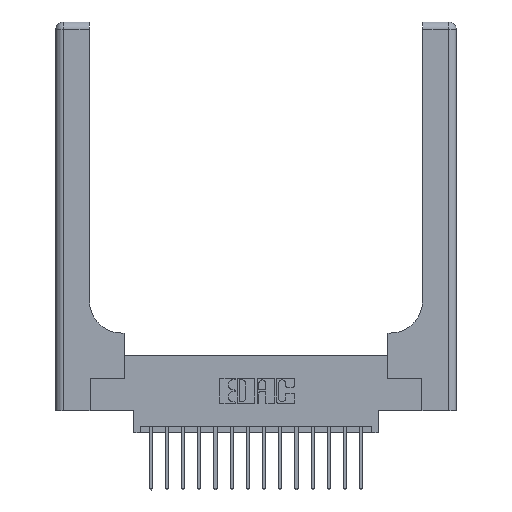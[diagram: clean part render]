
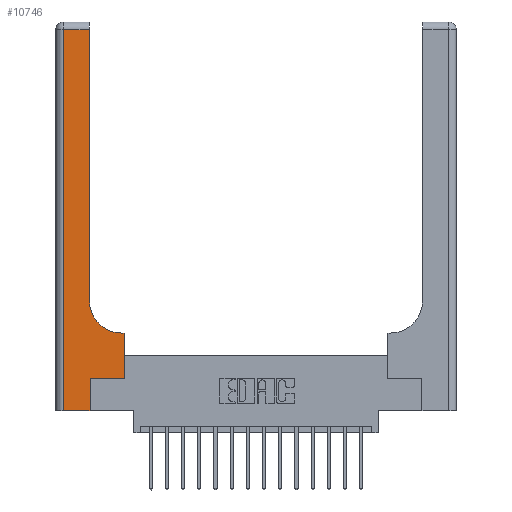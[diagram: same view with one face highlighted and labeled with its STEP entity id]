
A CAD part, top view. The second image highlights one B-rep face of the part: STEP entity #10746.
In plain terms, the highlighted planar face has unit normal (0, 0, 1).
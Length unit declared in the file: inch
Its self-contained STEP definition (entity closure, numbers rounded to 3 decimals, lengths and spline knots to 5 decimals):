
#49 = CARTESIAN_POINT ( 'NONE',  ( 0.06, 3., 0.37 ) ) ;
#151 = ORIENTED_EDGE ( 'NONE', *, *, #11037, .T. ) ;
#259 = LINE ( 'NONE', #7387, #7367 ) ;
#423 = CARTESIAN_POINT ( 'NONE',  ( 0.26, 2.94, 0.37 ) ) ;
#597 = LINE ( 'NONE', #11783, #11848 ) ;
#1410 = EDGE_CURVE ( 'NONE', #17213, #2887, #11189, .T. ) ;
#1603 = EDGE_CURVE ( 'NONE', #14179, #14640, #4391, .T. ) ;
#1753 = DIRECTION ( 'NONE',  ( -1., 0., 0. ) ) ;
#1934 = DIRECTION ( 'NONE',  ( 1., 0., 0. ) ) ;
#2081 = CARTESIAN_POINT ( 'NONE',  ( 0.06, 0., 0.37 ) ) ;
#2887 = VERTEX_POINT ( 'NONE', #10943 ) ;
#3300 = VECTOR ( 'NONE', #13908, 39.37008 ) ;
#3469 = ORIENTED_EDGE ( 'NONE', *, *, #1603, .T. ) ;
#3528 = CARTESIAN_POINT ( 'NONE',  ( 0.265, 0., 0.37 ) ) ;
#3656 = EDGE_LOOP ( 'NONE', ( #8706, #13283, #3469, #5011, #5250, #3946, #5719, #5957, #151 ) ) ;
#3802 = CARTESIAN_POINT ( 'NONE',  ( 0.51, 0.85, 0.37 ) ) ;
#3876 = VERTEX_POINT ( 'NONE', #10910 ) ;
#3946 = ORIENTED_EDGE ( 'NONE', *, *, #7716, .T. ) ;
#3948 = VECTOR ( 'NONE', #8976, 39.37008 ) ;
#4228 = DIRECTION ( 'NONE',  ( -1., 0., 0. ) ) ;
#4391 = LINE ( 'NONE', #49, #7697 ) ;
#4493 = AXIS2_PLACEMENT_3D ( 'NONE', #3802, #13614, #5221 ) ;
#5011 = ORIENTED_EDGE ( 'NONE', *, *, #11276, .T. ) ;
#5221 = DIRECTION ( 'NONE',  ( 1., 0., 0. ) ) ;
#5250 = ORIENTED_EDGE ( 'NONE', *, *, #1410, .T. ) ;
#5719 = ORIENTED_EDGE ( 'NONE', *, *, #7726, .T. ) ;
#5957 = ORIENTED_EDGE ( 'NONE', *, *, #18196, .T. ) ;
#5983 = CARTESIAN_POINT ( 'NONE',  ( 0., 3., 0.37 ) ) ;
#6732 = AXIS2_PLACEMENT_3D ( 'NONE', #5983, #15788, #7389 ) ;
#6751 = VECTOR ( 'NONE', #10928, 39.37008 ) ;
#6885 = VERTEX_POINT ( 'NONE', #10279 ) ;
#7297 = CARTESIAN_POINT ( 'NONE',  ( 0., 0., 0.37 ) ) ;
#7321 = PLANE ( 'NONE',  #6732 ) ;
#7367 = VECTOR ( 'NONE', #1753, 39.37008 ) ;
#7387 = CARTESIAN_POINT ( 'NONE',  ( 0., 2.94, 0.37 ) ) ;
#7389 = DIRECTION ( 'NONE',  ( -1., 0., 0. ) ) ;
#7697 = VECTOR ( 'NONE', #17817, 39.37008 ) ;
#7716 = EDGE_CURVE ( 'NONE', #2887, #3876, #597, .T. ) ;
#7726 = EDGE_CURVE ( 'NONE', #3876, #16120, #11396, .T. ) ;
#8358 = VERTEX_POINT ( 'NONE', #423 ) ;
#8706 = ORIENTED_EDGE ( 'NONE', *, *, #9185, .T. ) ;
#8719 = DIRECTION ( 'NONE',  ( 1., 0., 0. ) ) ;
#8976 = DIRECTION ( 'NONE',  ( 0., 1., 0. ) ) ;
#9185 = EDGE_CURVE ( 'NONE', #13386, #8358, #10896, .T. ) ;
#9306 = CIRCLE ( 'NONE', #4493, 0.25 ) ;
#9514 = LINE ( 'NONE', #7297, #16560 ) ;
#9520 = CARTESIAN_POINT ( 'NONE',  ( 0.26, 3., 0.37 ) ) ;
#9976 = FACE_OUTER_BOUND ( 'NONE', #3656, .T. ) ;
#10279 = CARTESIAN_POINT ( 'NONE',  ( 0.51, 0.6, 0.37 ) ) ;
#10746 = ADVANCED_FACE ( 'NONE', ( #9976 ), #7321, .F. ) ;
#10896 = LINE ( 'NONE', #9520, #6751 ) ;
#10910 = CARTESIAN_POINT ( 'NONE',  ( 0.528, 0.25, 0.37 ) ) ;
#10928 = DIRECTION ( 'NONE',  ( 0., 1., 0. ) ) ;
#10943 = CARTESIAN_POINT ( 'NONE',  ( 0.265, 0.25, 0.37 ) ) ;
#11037 = EDGE_CURVE ( 'NONE', #6885, #13386, #9306, .T. ) ;
#11189 = LINE ( 'NONE', #14123, #3300 ) ;
#11211 = CARTESIAN_POINT ( 'NONE',  ( 0.26, 0.6, 0.37 ) ) ;
#11276 = EDGE_CURVE ( 'NONE', #14640, #17213, #9514, .T. ) ;
#11396 = LINE ( 'NONE', #14613, #3948 ) ;
#11783 = CARTESIAN_POINT ( 'NONE',  ( 0.265, 0.25, 0.37 ) ) ;
#11848 = VECTOR ( 'NONE', #1934, 39.37008 ) ;
#12781 = VECTOR ( 'NONE', #4228, 39.37008 ) ;
#13283 = ORIENTED_EDGE ( 'NONE', *, *, #16157, .T. ) ;
#13386 = VERTEX_POINT ( 'NONE', #17262 ) ;
#13614 = DIRECTION ( 'NONE',  ( 0., 0., -1. ) ) ;
#13672 = LINE ( 'NONE', #11211, #12781 ) ;
#13908 = DIRECTION ( 'NONE',  ( 0., 1., 0. ) ) ;
#14123 = CARTESIAN_POINT ( 'NONE',  ( 0.265, 0., 0.37 ) ) ;
#14179 = VERTEX_POINT ( 'NONE', #16321 ) ;
#14613 = CARTESIAN_POINT ( 'NONE',  ( 0.528, 0.25, 0.37 ) ) ;
#14640 = VERTEX_POINT ( 'NONE', #2081 ) ;
#15735 = CARTESIAN_POINT ( 'NONE',  ( 0.528, 0.6, 0.37 ) ) ;
#15788 = DIRECTION ( 'NONE',  ( 0., 0., -1. ) ) ;
#16120 = VERTEX_POINT ( 'NONE', #15735 ) ;
#16157 = EDGE_CURVE ( 'NONE', #8358, #14179, #259, .T. ) ;
#16321 = CARTESIAN_POINT ( 'NONE',  ( 0.06, 2.94, 0.37 ) ) ;
#16560 = VECTOR ( 'NONE', #8719, 39.37008 ) ;
#17213 = VERTEX_POINT ( 'NONE', #3528 ) ;
#17262 = CARTESIAN_POINT ( 'NONE',  ( 0.26, 0.85, 0.37 ) ) ;
#17817 = DIRECTION ( 'NONE',  ( 0., -1., 0. ) ) ;
#18196 = EDGE_CURVE ( 'NONE', #16120, #6885, #13672, .T. ) ;
